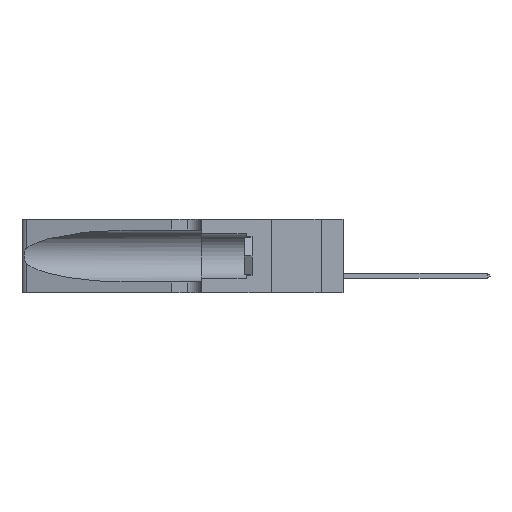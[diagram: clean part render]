
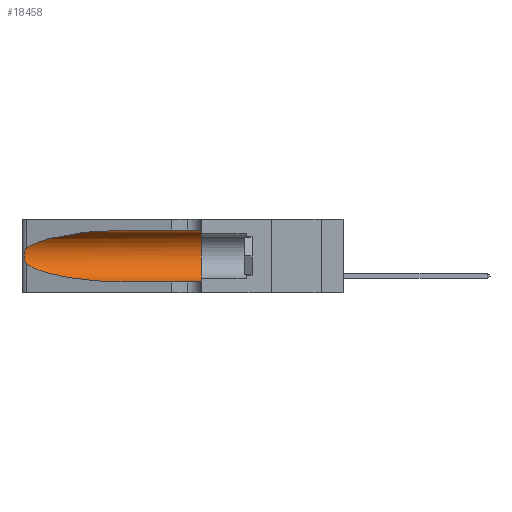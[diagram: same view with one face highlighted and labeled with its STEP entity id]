
A CAD part, left-side view. The second image highlights one B-rep face of the part: STEP entity #18458.
In plain terms, the highlighted cylindrical face has radius 3.308 mm (diameter 6.617 mm), a partial arc.
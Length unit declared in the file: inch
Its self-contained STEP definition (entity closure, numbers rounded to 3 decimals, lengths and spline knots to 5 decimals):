
#575 = ORIENTED_EDGE ( 'NONE', *, *, #38661, .T. ) ;
#1247 = CARTESIAN_POINT ( 'NONE',  ( 0.25487, 1.22718, 0.14631 ) ) ;
#1853 = VERTEX_POINT ( 'NONE', #7851 ) ;
#2436 = CARTESIAN_POINT ( 'NONE',  ( 0.18966, 0.96281, 0.05475 ) ) ;
#2674 = CARTESIAN_POINT ( 'NONE',  ( 0.25854, 1.2359, 0.20912 ) ) ;
#2823 = CARTESIAN_POINT ( 'NONE',  ( 0.26017, 1.23833, 0.17102 ) ) ;
#2835 = FACE_OUTER_BOUND ( 'NONE', #36723, .T. ) ;
#3062 = ORIENTED_EDGE ( 'NONE', *, *, #42222, .T. ) ;
#3890 = CARTESIAN_POINT ( 'NONE',  ( 0.1305, 0.35, 0.185 ) ) ;
#5347 = CARTESIAN_POINT ( 'NONE',  ( 0.1305, 0.35, 0.31525 ) ) ;
#5929 = VERTEX_POINT ( 'NONE', #47408 ) ;
#6503 = CARTESIAN_POINT ( 'NONE',  ( 0.26018, 1.23835, 0.19895 ) ) ;
#6670 = CARTESIAN_POINT ( 'NONE',  ( 0.25856, 1.23593, 0.16098 ) ) ;
#7851 = CARTESIAN_POINT ( 'NONE',  ( 0.1305, 0.72297, 0.05475 ) ) ;
#9280 = LINE ( 'NONE', #17604, #44535 ) ;
#9649 = CARTESIAN_POINT ( 'NONE',  ( 0.25487, 1.22718, 0.22369 ) ) ;
#9726 = DIRECTION ( 'NONE',  ( 0., -1., 0. ) ) ;
#11126 = DIRECTION ( 'NONE',  ( 0., 1., 0. ) ) ;
#12128 = CARTESIAN_POINT ( 'NONE',  ( 0.25487, 1.22718, 0.14631 ) ) ;
#12396 =( BOUNDED_CURVE ( )  B_SPLINE_CURVE ( 3, ( #13668, #28689, #32490, #9649 ),
 .UNSPECIFIED., .F., .F. ) 
 B_SPLINE_CURVE_WITH_KNOTS ( ( 4, 4 ),
 ( 1.5708, 2.84003 ),
 .UNSPECIFIED. ) 
 CURVE ( )  GEOMETRIC_REPRESENTATION_ITEM ( )  RATIONAL_B_SPLINE_CURVE ( ( 1., 0.87, 0.87, 1. ) ) 
 REPRESENTATION_ITEM ( '' )  );
#12857 = VERTEX_POINT ( 'NONE', #15720 ) ;
#13507 = CARTESIAN_POINT ( 'NONE',  ( 0.1305, 1.61858, 0.31525 ) ) ;
#13668 = CARTESIAN_POINT ( 'NONE',  ( 0.1305, 0.72297, 0.31525 ) ) ;
#15720 = CARTESIAN_POINT ( 'NONE',  ( 0.1305, 0.72297, 0.31525 ) ) ;
#15763 = LINE ( 'NONE', #13507, #38485 ) ;
#17544 = DIRECTION ( 'NONE',  ( 0., -1., 0. ) ) ;
#17604 = CARTESIAN_POINT ( 'NONE',  ( 0.1305, 1.61858, 0.05475 ) ) ;
#17813 = CARTESIAN_POINT ( 'NONE',  ( 0.25487, 1.22718, 0.14631 ) ) ;
#17865 = CARTESIAN_POINT ( 'NONE',  ( 0.25555, 1.22994, 0.2215 ) ) ;
#18307 = CARTESIAN_POINT ( 'NONE',  ( 0.2373, 1.15595, 0.08982 ) ) ;
#18458 = ADVANCED_FACE ( 'NONE', ( #2835 ), #30853, .F. ) ;
#20214 = AXIS2_PLACEMENT_3D ( 'NONE', #3890, #11126, #45756 ) ;
#21726 = CARTESIAN_POINT ( 'NONE',  ( 0.25639, 1.23184, 0.21858 ) ) ;
#22208 = CARTESIAN_POINT ( 'NONE',  ( 0.25555, 1.22993, 0.14849 ) ) ;
#25510 = CARTESIAN_POINT ( 'NONE',  ( 0.25487, 1.22718, 0.22369 ) ) ;
#26119 = ORIENTED_EDGE ( 'NONE', *, *, #30352, .F. ) ;
#27526 = DIRECTION ( 'NONE',  ( 0., 0., -1. ) ) ;
#28271 =( BOUNDED_CURVE ( )  B_SPLINE_CURVE ( 3, ( #17813, #18307, #2436, #40992 ),
 .UNSPECIFIED., .F., .F. ) 
 B_SPLINE_CURVE_WITH_KNOTS ( ( 4, 4 ),
 ( 3.44316, 4.71239 ),
 .UNSPECIFIED. ) 
 CURVE ( )  GEOMETRIC_REPRESENTATION_ITEM ( )  RATIONAL_B_SPLINE_CURVE ( ( 1., 0.87, 0.87, 1. ) ) 
 REPRESENTATION_ITEM ( '' )  );
#28689 = CARTESIAN_POINT ( 'NONE',  ( 0.18966, 0.96281, 0.31525 ) ) ;
#29199 = CARTESIAN_POINT ( 'NONE',  ( 0.26075, 1.23896, 0.178 ) ) ;
#29525 = CARTESIAN_POINT ( 'NONE',  ( 0.25787, 1.23484, 0.2124 ) ) ;
#30352 = EDGE_CURVE ( 'NONE', #12857, #41338, #15763, .T. ) ;
#30840 = CIRCLE ( 'NONE', #20214, 0.13025 ) ;
#30853 = CYLINDRICAL_SURFACE ( 'NONE', #45513, 0.13025 ) ;
#31368 = DIRECTION ( 'NONE',  ( 0., -1., 0. ) ) ;
#32490 = CARTESIAN_POINT ( 'NONE',  ( 0.2373, 1.15595, 0.28018 ) ) ;
#33152 = VERTEX_POINT ( 'NONE', #38410 ) ;
#33205 = CARTESIAN_POINT ( 'NONE',  ( 0.26075, 1.23896, 0.19203 ) ) ;
#34971 = EDGE_CURVE ( 'NONE', #12857, #33152, #12396, .T. ) ;
#36723 = EDGE_LOOP ( 'NONE', ( #43188, #3062, #575, #45416, #48598, #26119 ) ) ;
#38410 = CARTESIAN_POINT ( 'NONE',  ( 0.25487, 1.22718, 0.22369 ) ) ;
#38485 = VECTOR ( 'NONE', #17544, 39.37008 ) ;
#38661 = EDGE_CURVE ( 'NONE', #42473, #1853, #28271, .T. ) ;
#39224 = CARTESIAN_POINT ( 'NONE',  ( 0.1305, 1.61858, 0.185 ) ) ;
#39283 = B_SPLINE_CURVE_WITH_KNOTS ( 'NONE', 3,
 ( #25510, #17865, #21726, #29525, #2674, #6503, #33205, #29199, #2823, #6670, #48663, #41202, #22208, #12128 ),
 .UNSPECIFIED., .F., .F.,
 ( 4, 2, 2, 2, 2, 2, 4 ),
 ( 0., 0.00027, 0.00053, 0.00107, 0.0016, 0.00187, 0.00214 ),
 .UNSPECIFIED. ) ;
#40992 = CARTESIAN_POINT ( 'NONE',  ( 0.1305, 0.72297, 0.05475 ) ) ;
#41038 = EDGE_CURVE ( 'NONE', #41338, #5929, #30840, .T. ) ;
#41202 = CARTESIAN_POINT ( 'NONE',  ( 0.25639, 1.23186, 0.15144 ) ) ;
#41338 = VERTEX_POINT ( 'NONE', #5347 ) ;
#41530 = EDGE_CURVE ( 'NONE', #1853, #5929, #9280, .T. ) ;
#42222 = EDGE_CURVE ( 'NONE', #33152, #42473, #39283, .T. ) ;
#42473 = VERTEX_POINT ( 'NONE', #1247 ) ;
#43188 = ORIENTED_EDGE ( 'NONE', *, *, #34971, .T. ) ;
#44535 = VECTOR ( 'NONE', #9726, 39.37008 ) ;
#45416 = ORIENTED_EDGE ( 'NONE', *, *, #41530, .T. ) ;
#45513 = AXIS2_PLACEMENT_3D ( 'NONE', #39224, #31368, #27526 ) ;
#45756 = DIRECTION ( 'NONE',  ( 0., 0., 1. ) ) ;
#47408 = CARTESIAN_POINT ( 'NONE',  ( 0.1305, 0.35, 0.05475 ) ) ;
#48598 = ORIENTED_EDGE ( 'NONE', *, *, #41038, .F. ) ;
#48663 = CARTESIAN_POINT ( 'NONE',  ( 0.25789, 1.23486, 0.15765 ) ) ;
